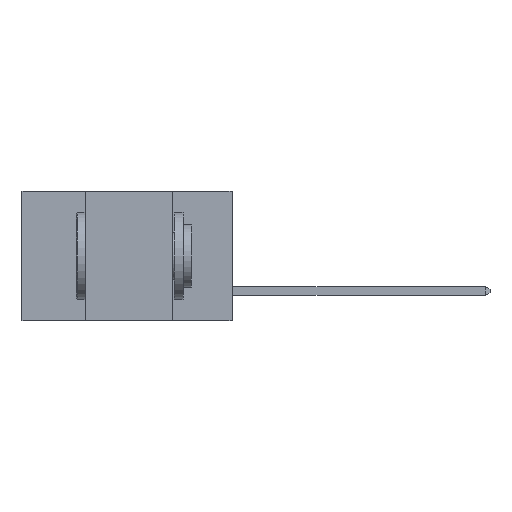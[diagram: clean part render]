
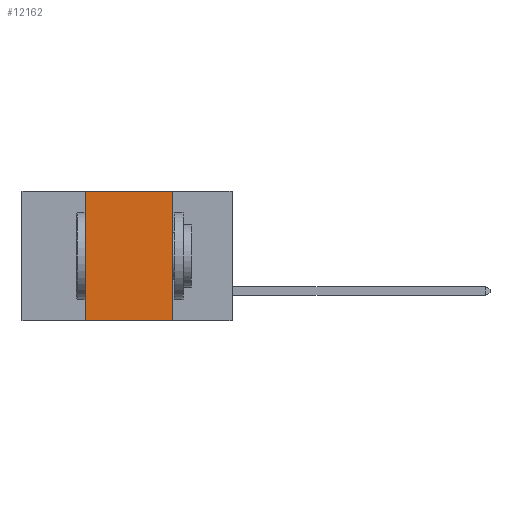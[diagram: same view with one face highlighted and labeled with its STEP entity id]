
A CAD part, left-side view. The second image highlights one B-rep face of the part: STEP entity #12162.
In plain terms, the highlighted planar face has unit normal (-1, 0, 0).
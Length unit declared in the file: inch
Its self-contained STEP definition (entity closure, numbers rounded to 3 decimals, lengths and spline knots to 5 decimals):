
#853 = EDGE_CURVE ( 'NONE', #31508, #19436, #36584, .T. ) ;
#1644 = EDGE_CURVE ( 'NONE', #27007, #14328, #7310, .T. ) ;
#5161 = DIRECTION ( 'NONE',  ( 0., 0., -1. ) ) ;
#6957 = DIRECTION ( 'NONE',  ( 0., 0., -1. ) ) ;
#7310 = LINE ( 'NONE', #32584, #31264 ) ;
#7434 = ORIENTED_EDGE ( 'NONE', *, *, #30797, .F. ) ;
#7478 = VECTOR ( 'NONE', #9002, 39.37008 ) ;
#8351 = CARTESIAN_POINT ( 'NONE',  ( 0., 0.17, 0. ) ) ;
#9002 = DIRECTION ( 'NONE',  ( 0., -1., 0. ) ) ;
#9929 = CARTESIAN_POINT ( 'NONE',  ( 0., 0.42, -0.37 ) ) ;
#10338 = EDGE_LOOP ( 'NONE', ( #23159, #7434, #34269, #12887 ) ) ;
#11007 = EDGE_CURVE ( 'NONE', #27007, #19436, #30523, .T. ) ;
#11873 = FACE_OUTER_BOUND ( 'NONE', #10338, .T. ) ;
#12162 = ADVANCED_FACE ( 'NONE', ( #11873 ), #39303, .F. ) ;
#12789 = AXIS2_PLACEMENT_3D ( 'NONE', #20811, #24003, #5161 ) ;
#12887 = ORIENTED_EDGE ( 'NONE', *, *, #11007, .T. ) ;
#14328 = VERTEX_POINT ( 'NONE', #34195 ) ;
#14885 = CARTESIAN_POINT ( 'NONE',  ( 0., 0.6, -0.37 ) ) ;
#18077 = DIRECTION ( 'NONE',  ( 0., -1., 0. ) ) ;
#18311 = CARTESIAN_POINT ( 'NONE',  ( 0., 0.17, -0.37 ) ) ;
#18670 = CARTESIAN_POINT ( 'NONE',  ( 0., 0.17, 0. ) ) ;
#19436 = VERTEX_POINT ( 'NONE', #18311 ) ;
#20811 = CARTESIAN_POINT ( 'NONE',  ( 0., 0.6, 0. ) ) ;
#23159 = ORIENTED_EDGE ( 'NONE', *, *, #853, .F. ) ;
#24003 = DIRECTION ( 'NONE',  ( 1., 0., 0. ) ) ;
#27007 = VERTEX_POINT ( 'NONE', #9929 ) ;
#28429 = VECTOR ( 'NONE', #6957, 39.37008 ) ;
#30523 = LINE ( 'NONE', #14885, #36745 ) ;
#30797 = EDGE_CURVE ( 'NONE', #14328, #31508, #33355, .T. ) ;
#31264 = VECTOR ( 'NONE', #32319, 39.37008 ) ;
#31508 = VERTEX_POINT ( 'NONE', #18670 ) ;
#32319 = DIRECTION ( 'NONE',  ( 0., 0., 1. ) ) ;
#32584 = CARTESIAN_POINT ( 'NONE',  ( 0., 0.42, 0. ) ) ;
#33355 = LINE ( 'NONE', #39879, #7478 ) ;
#34195 = CARTESIAN_POINT ( 'NONE',  ( 0., 0.42, 0. ) ) ;
#34269 = ORIENTED_EDGE ( 'NONE', *, *, #1644, .F. ) ;
#36584 = LINE ( 'NONE', #8351, #28429 ) ;
#36745 = VECTOR ( 'NONE', #18077, 39.37008 ) ;
#39303 = PLANE ( 'NONE',  #12789 ) ;
#39879 = CARTESIAN_POINT ( 'NONE',  ( 0., 0.6, 0. ) ) ;
